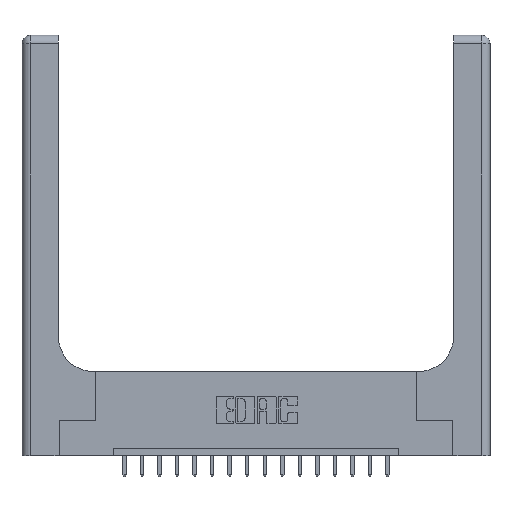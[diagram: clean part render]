
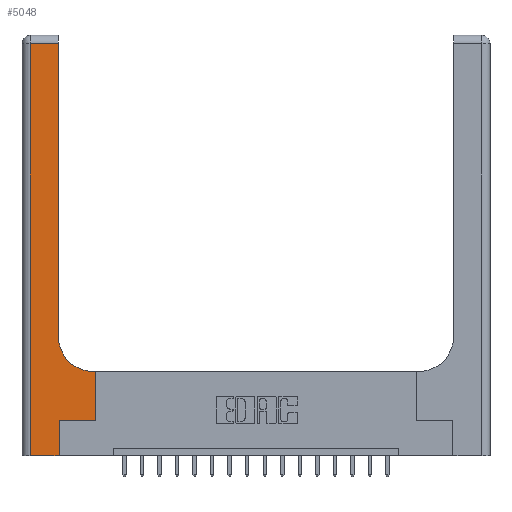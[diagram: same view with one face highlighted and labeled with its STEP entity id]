
A CAD part, top view. The second image highlights one B-rep face of the part: STEP entity #5048.
In plain terms, the highlighted planar face has unit normal (0, 0, 1).
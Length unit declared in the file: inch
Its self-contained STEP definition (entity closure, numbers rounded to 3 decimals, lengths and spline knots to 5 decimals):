
#150 = CARTESIAN_POINT ( 'NONE',  ( 0.528, 0.6, 0.37 ) ) ;
#1598 = LINE ( 'NONE', #13027, #6120 ) ;
#1764 = VERTEX_POINT ( 'NONE', #12991 ) ;
#1855 = VERTEX_POINT ( 'NONE', #150 ) ;
#1900 = VERTEX_POINT ( 'NONE', #3257 ) ;
#2023 = EDGE_CURVE ( 'NONE', #3923, #1855, #3677, .T. ) ;
#2302 = EDGE_CURVE ( 'NONE', #1764, #1900, #18501, .T. ) ;
#2500 = ORIENTED_EDGE ( 'NONE', *, *, #9856, .T. ) ;
#2557 = CARTESIAN_POINT ( 'NONE',  ( 0.528, 0.25, 0.37 ) ) ;
#2856 = CARTESIAN_POINT ( 'NONE',  ( 0., 3., 0.37 ) ) ;
#2968 = VECTOR ( 'NONE', #18583, 39.37008 ) ;
#3257 = CARTESIAN_POINT ( 'NONE',  ( 0.06, 0., 0.37 ) ) ;
#3677 = LINE ( 'NONE', #2557, #17592 ) ;
#3923 = VERTEX_POINT ( 'NONE', #15100 ) ;
#3928 = VERTEX_POINT ( 'NONE', #5555 ) ;
#4540 = EDGE_LOOP ( 'NONE', ( #9378, #2500, #8319, #12295, #10046, #11810, #6134, #16589, #12460 ) ) ;
#4854 = DIRECTION ( 'NONE',  ( 0., 1., 0. ) ) ;
#5048 = ADVANCED_FACE ( 'NONE', ( #5135 ), #9764, .F. ) ;
#5135 = FACE_OUTER_BOUND ( 'NONE', #4540, .T. ) ;
#5452 = DIRECTION ( 'NONE',  ( 0., 0., -1. ) ) ;
#5555 = CARTESIAN_POINT ( 'NONE',  ( 0.265, 0., 0.37 ) ) ;
#6120 = VECTOR ( 'NONE', #14803, 39.37008 ) ;
#6134 = ORIENTED_EDGE ( 'NONE', *, *, #2023, .T. ) ;
#6576 = VERTEX_POINT ( 'NONE', #9061 ) ;
#6610 = LINE ( 'NONE', #13565, #14726 ) ;
#7248 = VERTEX_POINT ( 'NONE', #10261 ) ;
#7284 = DIRECTION ( 'NONE',  ( -1., 0., 0. ) ) ;
#8016 = VERTEX_POINT ( 'NONE', #10158 ) ;
#8102 = DIRECTION ( 'NONE',  ( 0., -1., 0. ) ) ;
#8218 = DIRECTION ( 'NONE',  ( 1., 0., 0. ) ) ;
#8319 = ORIENTED_EDGE ( 'NONE', *, *, #2302, .T. ) ;
#9061 = CARTESIAN_POINT ( 'NONE',  ( 0.51, 0.6, 0.37 ) ) ;
#9069 = EDGE_CURVE ( 'NONE', #6576, #8016, #9568, .T. ) ;
#9378 = ORIENTED_EDGE ( 'NONE', *, *, #14403, .T. ) ;
#9568 = CIRCLE ( 'NONE', #13127, 0.25 ) ;
#9764 = PLANE ( 'NONE',  #14041 ) ;
#9856 = EDGE_CURVE ( 'NONE', #7248, #1764, #1598, .T. ) ;
#10046 = ORIENTED_EDGE ( 'NONE', *, *, #18588, .T. ) ;
#10158 = CARTESIAN_POINT ( 'NONE',  ( 0.26, 0.85, 0.37 ) ) ;
#10261 = CARTESIAN_POINT ( 'NONE',  ( 0.26, 2.94, 0.37 ) ) ;
#10478 = EDGE_CURVE ( 'NONE', #13623, #3923, #11760, .T. ) ;
#10725 = CARTESIAN_POINT ( 'NONE',  ( 0.06, 3., 0.37 ) ) ;
#11302 = VECTOR ( 'NONE', #8218, 39.37008 ) ;
#11760 = LINE ( 'NONE', #15309, #11302 ) ;
#11810 = ORIENTED_EDGE ( 'NONE', *, *, #10478, .T. ) ;
#12295 = ORIENTED_EDGE ( 'NONE', *, *, #13360, .T. ) ;
#12460 = ORIENTED_EDGE ( 'NONE', *, *, #9069, .T. ) ;
#12562 = DIRECTION ( 'NONE',  ( 1., 0., 0. ) ) ;
#12780 = DIRECTION ( 'NONE',  ( 0., 1., 0. ) ) ;
#12991 = CARTESIAN_POINT ( 'NONE',  ( 0.06, 2.94, 0.37 ) ) ;
#13027 = CARTESIAN_POINT ( 'NONE',  ( 0., 2.94, 0.37 ) ) ;
#13064 = CARTESIAN_POINT ( 'NONE',  ( 0.26, 0.6, 0.37 ) ) ;
#13127 = AXIS2_PLACEMENT_3D ( 'NONE', #15580, #18435, #14267 ) ;
#13360 = EDGE_CURVE ( 'NONE', #1900, #3928, #13454, .T. ) ;
#13454 = LINE ( 'NONE', #18400, #15885 ) ;
#13565 = CARTESIAN_POINT ( 'NONE',  ( 0.265, 0., 0.37 ) ) ;
#13623 = VERTEX_POINT ( 'NONE', #18200 ) ;
#14041 = AXIS2_PLACEMENT_3D ( 'NONE', #2856, #5452, #7284 ) ;
#14267 = DIRECTION ( 'NONE',  ( 1., 0., 0. ) ) ;
#14403 = EDGE_CURVE ( 'NONE', #8016, #7248, #15662, .T. ) ;
#14726 = VECTOR ( 'NONE', #4854, 39.37008 ) ;
#14755 = VECTOR ( 'NONE', #12780, 39.37008 ) ;
#14803 = DIRECTION ( 'NONE',  ( -1., 0., 0. ) ) ;
#15100 = CARTESIAN_POINT ( 'NONE',  ( 0.528, 0.25, 0.37 ) ) ;
#15128 = DIRECTION ( 'NONE',  ( 0., 1., 0. ) ) ;
#15309 = CARTESIAN_POINT ( 'NONE',  ( 0.265, 0.25, 0.37 ) ) ;
#15580 = CARTESIAN_POINT ( 'NONE',  ( 0.51, 0.85, 0.37 ) ) ;
#15581 = CARTESIAN_POINT ( 'NONE',  ( 0.26, 3., 0.37 ) ) ;
#15662 = LINE ( 'NONE', #15581, #14755 ) ;
#15885 = VECTOR ( 'NONE', #12562, 39.37008 ) ;
#16054 = VECTOR ( 'NONE', #8102, 39.37008 ) ;
#16372 = EDGE_CURVE ( 'NONE', #1855, #6576, #16442, .T. ) ;
#16442 = LINE ( 'NONE', #13064, #2968 ) ;
#16589 = ORIENTED_EDGE ( 'NONE', *, *, #16372, .T. ) ;
#17592 = VECTOR ( 'NONE', #15128, 39.37008 ) ;
#18200 = CARTESIAN_POINT ( 'NONE',  ( 0.265, 0.25, 0.37 ) ) ;
#18400 = CARTESIAN_POINT ( 'NONE',  ( 0., 0., 0.37 ) ) ;
#18435 = DIRECTION ( 'NONE',  ( 0., 0., -1. ) ) ;
#18501 = LINE ( 'NONE', #10725, #16054 ) ;
#18583 = DIRECTION ( 'NONE',  ( -1., 0., 0. ) ) ;
#18588 = EDGE_CURVE ( 'NONE', #3928, #13623, #6610, .T. ) ;
